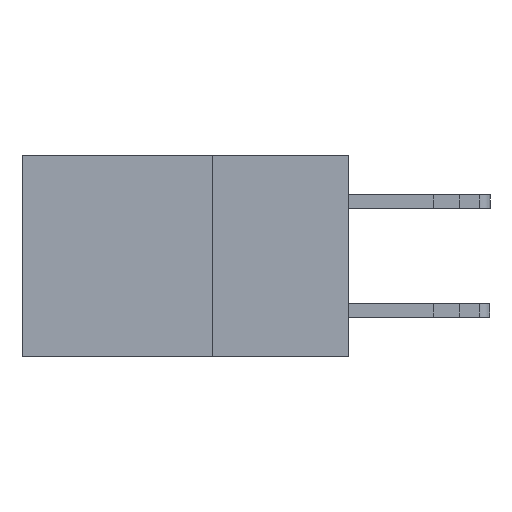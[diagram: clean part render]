
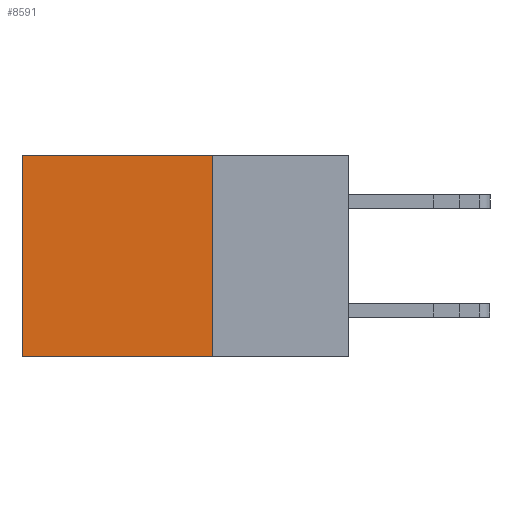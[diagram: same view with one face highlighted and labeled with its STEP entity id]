
A CAD part, left-side view. The second image highlights one B-rep face of the part: STEP entity #8591.
In plain terms, the highlighted planar face has unit normal (-1, 0, 0).
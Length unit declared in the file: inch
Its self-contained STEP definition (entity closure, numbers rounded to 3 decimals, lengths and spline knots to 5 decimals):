
#395 = DIRECTION ( 'NONE',  ( 0., 1., 0. ) ) ;
#757 = VECTOR ( 'NONE', #7292, 39.37008 ) ;
#1740 = LINE ( 'NONE', #15248, #10305 ) ;
#2040 = CARTESIAN_POINT ( 'NONE',  ( 0.298, 0.6, 0. ) ) ;
#4661 = FACE_OUTER_BOUND ( 'NONE', #9926, .T. ) ;
#4700 = VERTEX_POINT ( 'NONE', #9056 ) ;
#4991 = ORIENTED_EDGE ( 'NONE', *, *, #15331, .F. ) ;
#5351 = CARTESIAN_POINT ( 'NONE',  ( 0.298, 0.25, -0.37 ) ) ;
#5505 = DIRECTION ( 'NONE',  ( 0., 0., -1. ) ) ;
#5901 = DIRECTION ( 'NONE',  ( 1., 0., 0. ) ) ;
#6260 = CARTESIAN_POINT ( 'NONE',  ( 0.298, 0.6, 0. ) ) ;
#7292 = DIRECTION ( 'NONE',  ( 0., 0., -1. ) ) ;
#7426 = VECTOR ( 'NONE', #5505, 39.37008 ) ;
#7877 = ORIENTED_EDGE ( 'NONE', *, *, #18800, .T. ) ;
#8591 = ADVANCED_FACE ( 'NONE', ( #4661 ), #16215, .F. ) ;
#9056 = CARTESIAN_POINT ( 'NONE',  ( 0.298, 0.25, 0. ) ) ;
#9862 = LINE ( 'NONE', #10704, #757 ) ;
#9926 = EDGE_LOOP ( 'NONE', ( #7877, #4991, #22080, #17395 ) ) ;
#10305 = VECTOR ( 'NONE', #13550, 39.37008 ) ;
#10704 = CARTESIAN_POINT ( 'NONE',  ( 0.298, 0.25, 0. ) ) ;
#12501 = LINE ( 'NONE', #2040, #7426 ) ;
#12518 = VERTEX_POINT ( 'NONE', #6260 ) ;
#12760 = LINE ( 'NONE', #17591, #16855 ) ;
#12925 = EDGE_CURVE ( 'NONE', #4700, #15933, #9862, .T. ) ;
#13550 = DIRECTION ( 'NONE',  ( 0., 1., 0. ) ) ;
#13871 = CARTESIAN_POINT ( 'NONE',  ( 0.298, 0.6, -0.37 ) ) ;
#15248 = CARTESIAN_POINT ( 'NONE',  ( 0.298, 0.25, 0. ) ) ;
#15331 = EDGE_CURVE ( 'NONE', #15933, #16462, #12760, .T. ) ;
#15933 = VERTEX_POINT ( 'NONE', #5351 ) ;
#16215 = PLANE ( 'NONE',  #21588 ) ;
#16462 = VERTEX_POINT ( 'NONE', #13871 ) ;
#16855 = VECTOR ( 'NONE', #395, 39.37008 ) ;
#17395 = ORIENTED_EDGE ( 'NONE', *, *, #19278, .T. ) ;
#17591 = CARTESIAN_POINT ( 'NONE',  ( 0.298, 0.25, -0.37 ) ) ;
#17954 = DIRECTION ( 'NONE',  ( 0., 0., -1. ) ) ;
#18800 = EDGE_CURVE ( 'NONE', #12518, #16462, #12501, .T. ) ;
#19278 = EDGE_CURVE ( 'NONE', #4700, #12518, #1740, .T. ) ;
#21238 = CARTESIAN_POINT ( 'NONE',  ( 0.298, 0.25, 0. ) ) ;
#21588 = AXIS2_PLACEMENT_3D ( 'NONE', #21238, #5901, #17954 ) ;
#22080 = ORIENTED_EDGE ( 'NONE', *, *, #12925, .F. ) ;
